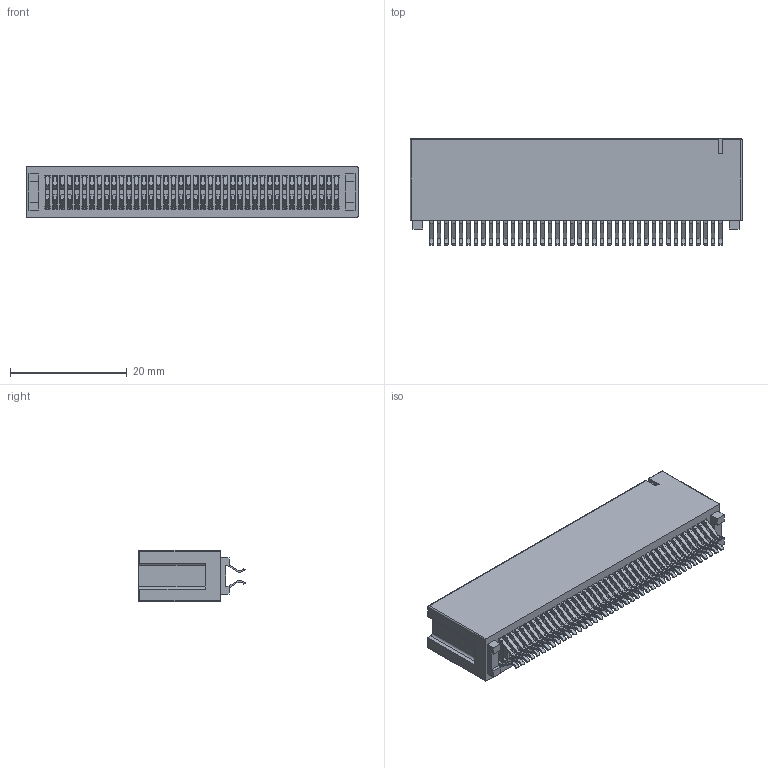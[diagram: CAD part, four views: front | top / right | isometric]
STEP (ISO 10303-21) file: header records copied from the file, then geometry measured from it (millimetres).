
FILE_DESCRIPTION (( 'STEP AP203' ), '1' );
FILE_NAME ('302-080-256-201.STEP', '2024-04-06T14:33:22', ( '' ), ( '' ), 'SwSTEP 2.0', 'SolidWorks 2023', '' );
FILE_SCHEMA (( 'CONFIG_CONTROL_DESIGN' ));
Length unit declared in the file: millimetre
Products named in the file (3): HSG_Vertical HSG; 302-080-256-201; Contact_302-290-X56
Assembly tree (81 placements, depth 2):
  302-080-256-201
    HSG_Vertical HSG
    Contact_302-290-X56  x80
Bounding box: 56.9 x 18.3 x 8.88 mm (x, y, z)
Volume: 4408 mm3; surface area: 12310.9 mm2
Topology: 81 solids, 81 shells, 3866 faces, 11528 edges, 7624 vertices
Faces by surface type: plane 2569, cylinder 1293, sphere 4
Entity records: 31095 total; most frequent: ORIENTED_EDGE 5352, CARTESIAN_POINT 5264, DIRECTION 4306, EDGE_CURVE 2676, LINE 2618, VECTOR 2618, VERTEX_POINT 1778, AXIS2_PLACEMENT_3D 844
